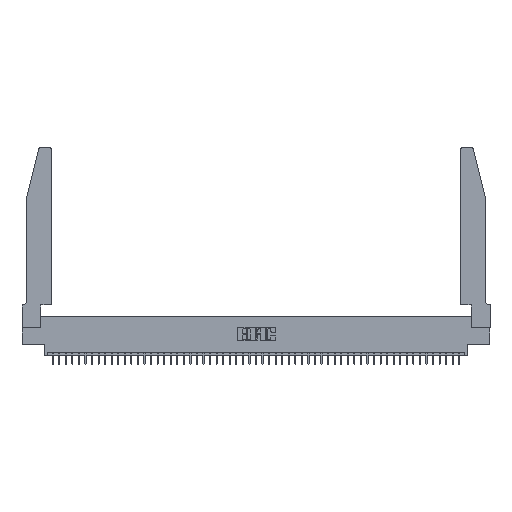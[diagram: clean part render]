
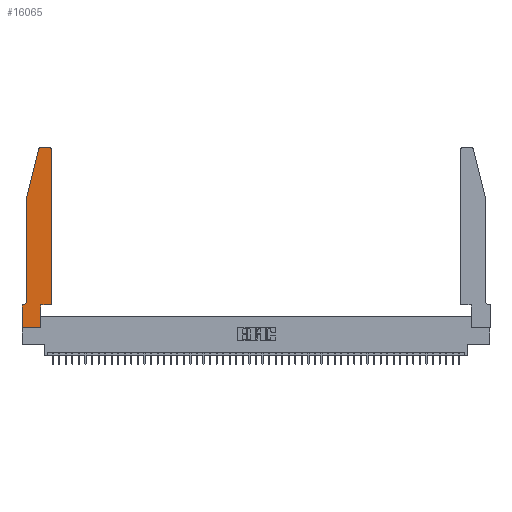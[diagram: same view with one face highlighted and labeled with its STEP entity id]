
A CAD part, top view. The second image highlights one B-rep face of the part: STEP entity #16065.
In plain terms, the highlighted planar face has unit normal (0, 0, 1).
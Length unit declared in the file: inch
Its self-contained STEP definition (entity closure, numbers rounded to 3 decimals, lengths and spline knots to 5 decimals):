
#1012 = CARTESIAN_POINT ( 'NONE',  ( 0.2865, 0., 0.37 ) ) ;
#1085 = ORIENTED_EDGE ( 'NONE', *, *, #47904, .T. ) ;
#1101 = VERTEX_POINT ( 'NONE', #1012 ) ;
#1142 = VECTOR ( 'NONE', #15414, 39.37008 ) ;
#1398 = DIRECTION ( 'NONE',  ( 1., 0., 0. ) ) ;
#1459 = CARTESIAN_POINT ( 'NONE',  ( 0.0755, 0.42, 0.37 ) ) ;
#1651 = CARTESIAN_POINT ( 'NONE',  ( 0.4505, 0.35, 0.37 ) ) ;
#1958 = EDGE_CURVE ( 'NONE', #10670, #44794, #8432, .T. ) ;
#1998 = CARTESIAN_POINT ( 'NONE',  ( 0., 0.35, 0.37 ) ) ;
#2457 = VERTEX_POINT ( 'NONE', #13750 ) ;
#3552 = CIRCLE ( 'NONE', #33524, 0.03 ) ;
#5090 = ORIENTED_EDGE ( 'NONE', *, *, #23087, .T. ) ;
#5956 = AXIS2_PLACEMENT_3D ( 'NONE', #39325, #47918, #23639 ) ;
#6470 = DIRECTION ( 'NONE',  ( 1., 0., 0. ) ) ;
#8432 = CIRCLE ( 'NONE', #5956, 0.07 ) ;
#8491 = LINE ( 'NONE', #9011, #38162 ) ;
#8721 = VECTOR ( 'NONE', #43241, 39.37008 ) ;
#9011 = CARTESIAN_POINT ( 'NONE',  ( 0.2865, 0.35, 0.37 ) ) ;
#9894 = EDGE_CURVE ( 'NONE', #2457, #12290, #41487, .T. ) ;
#10603 = LINE ( 'NONE', #13733, #8721 ) ;
#10623 = CARTESIAN_POINT ( 'NONE',  ( 0.0055, 0.35, 0.37 ) ) ;
#10670 = VERTEX_POINT ( 'NONE', #1459 ) ;
#10853 = VERTEX_POINT ( 'NONE', #34338 ) ;
#11432 = DIRECTION ( 'NONE',  ( 0., 0., 1. ) ) ;
#12290 = VERTEX_POINT ( 'NONE', #39814 ) ;
#12428 = LINE ( 'NONE', #24182, #37198 ) ;
#13638 = EDGE_CURVE ( 'NONE', #48304, #2457, #26218, .T. ) ;
#13733 = CARTESIAN_POINT ( 'NONE',  ( 0.0755, 0.35, 0.37 ) ) ;
#13750 = CARTESIAN_POINT ( 'NONE',  ( 0.4205, 2.75, 0.37 ) ) ;
#13987 = CARTESIAN_POINT ( 'NONE',  ( 0.0755, 2., 0.37 ) ) ;
#14022 = LINE ( 'NONE', #45903, #24774 ) ;
#14073 = VECTOR ( 'NONE', #1398, 39.37008 ) ;
#14960 = DIRECTION ( 'NONE',  ( 1., 0., 0. ) ) ;
#15414 = DIRECTION ( 'NONE',  ( 0., 1., 0. ) ) ;
#15603 = EDGE_CURVE ( 'NONE', #25376, #17163, #29401, .T. ) ;
#15662 = VERTEX_POINT ( 'NONE', #1998 ) ;
#15694 = EDGE_CURVE ( 'NONE', #44794, #15662, #10603, .T. ) ;
#16065 = ADVANCED_FACE ( 'NONE', ( #51011 ), #35059, .T. ) ;
#17163 = VERTEX_POINT ( 'NONE', #47922 ) ;
#17617 = ORIENTED_EDGE ( 'NONE', *, *, #15694, .T. ) ;
#17690 = ORIENTED_EDGE ( 'NONE', *, *, #28602, .T. ) ;
#18051 = VERTEX_POINT ( 'NONE', #48573 ) ;
#18813 = ORIENTED_EDGE ( 'NONE', *, *, #30267, .T. ) ;
#20901 = CARTESIAN_POINT ( 'NONE',  ( 0.25487, 2.72718, 0.37 ) ) ;
#21481 = EDGE_CURVE ( 'NONE', #50397, #18051, #45545, .T. ) ;
#22804 = CARTESIAN_POINT ( 'NONE',  ( 0., 0.35, 0.37 ) ) ;
#23087 = EDGE_CURVE ( 'NONE', #15662, #10853, #49726, .T. ) ;
#23639 = DIRECTION ( 'NONE',  ( -1., 0., 0. ) ) ;
#24182 = CARTESIAN_POINT ( 'NONE',  ( 0.0755, 2., 0.37 ) ) ;
#24774 = VECTOR ( 'NONE', #6470, 39.37008 ) ;
#24789 = ORIENTED_EDGE ( 'NONE', *, *, #13638, .T. ) ;
#25048 = ORIENTED_EDGE ( 'NONE', *, *, #47272, .T. ) ;
#25376 = VERTEX_POINT ( 'NONE', #20901 ) ;
#26218 = CIRCLE ( 'NONE', #50425, 0.03 ) ;
#26321 = CARTESIAN_POINT ( 'NONE',  ( 0.2605, 2.75, 0.37 ) ) ;
#28602 = EDGE_CURVE ( 'NONE', #12290, #25376, #3552, .T. ) ;
#29401 = LINE ( 'NONE', #13987, #33845 ) ;
#30267 = EDGE_CURVE ( 'NONE', #18051, #48304, #43903, .T. ) ;
#32164 = ORIENTED_EDGE ( 'NONE', *, *, #15603, .T. ) ;
#32226 = ORIENTED_EDGE ( 'NONE', *, *, #1958, .T. ) ;
#33518 = DIRECTION ( 'NONE',  ( 0., -1., 0. ) ) ;
#33524 = AXIS2_PLACEMENT_3D ( 'NONE', #38479, #34797, #37692 ) ;
#33845 = VECTOR ( 'NONE', #45611, 39.37008 ) ;
#34338 = CARTESIAN_POINT ( 'NONE',  ( 0., 0., 0.37 ) ) ;
#34670 = EDGE_LOOP ( 'NONE', ( #38746, #17690, #32164, #51001, #32226, #17617, #5090, #25048, #1085, #42284, #18813, #24789 ) ) ;
#34797 = DIRECTION ( 'NONE',  ( 0., 0., 1. ) ) ;
#34963 = VECTOR ( 'NONE', #33518, 39.37008 ) ;
#35059 = PLANE ( 'NONE',  #47213 ) ;
#35426 = DIRECTION ( 'NONE',  ( 0., -1., 0. ) ) ;
#37198 = VECTOR ( 'NONE', #35426, 39.37008 ) ;
#37291 = DIRECTION ( 'NONE',  ( -1., 0., 0. ) ) ;
#37692 = DIRECTION ( 'NONE',  ( 1., 0., 0. ) ) ;
#38162 = VECTOR ( 'NONE', #45064, 39.37008 ) ;
#38479 = CARTESIAN_POINT ( 'NONE',  ( 0.284, 2.72, 0.37 ) ) ;
#38746 = ORIENTED_EDGE ( 'NONE', *, *, #9894, .T. ) ;
#38997 = DIRECTION ( 'NONE',  ( 0., 0., 1. ) ) ;
#39325 = CARTESIAN_POINT ( 'NONE',  ( 0.0055, 0.42, 0.37 ) ) ;
#39814 = CARTESIAN_POINT ( 'NONE',  ( 0.284, 2.75, 0.37 ) ) ;
#39860 = CARTESIAN_POINT ( 'NONE',  ( 0.2865, 0.35, 0.37 ) ) ;
#41487 = LINE ( 'NONE', #26321, #41814 ) ;
#41814 = VECTOR ( 'NONE', #37291, 39.37008 ) ;
#42284 = ORIENTED_EDGE ( 'NONE', *, *, #21481, .T. ) ;
#43241 = DIRECTION ( 'NONE',  ( -1., 0., 0. ) ) ;
#43676 = EDGE_CURVE ( 'NONE', #17163, #10670, #12428, .T. ) ;
#43903 = LINE ( 'NONE', #50949, #1142 ) ;
#44794 = VERTEX_POINT ( 'NONE', #10623 ) ;
#44798 = CARTESIAN_POINT ( 'NONE',  ( 0., 0., 0.37 ) ) ;
#45064 = DIRECTION ( 'NONE',  ( 0., 1., 0. ) ) ;
#45545 = LINE ( 'NONE', #1651, #14073 ) ;
#45611 = DIRECTION ( 'NONE',  ( -0.239, -0.971, 0. ) ) ;
#45903 = CARTESIAN_POINT ( 'NONE',  ( 0., 0., 0.37 ) ) ;
#47213 = AXIS2_PLACEMENT_3D ( 'NONE', #22804, #38997, #14960 ) ;
#47218 = CARTESIAN_POINT ( 'NONE',  ( 0.4205, 2.72, 0.37 ) ) ;
#47272 = EDGE_CURVE ( 'NONE', #10853, #1101, #14022, .T. ) ;
#47722 = DIRECTION ( 'NONE',  ( 1., 0., 0. ) ) ;
#47904 = EDGE_CURVE ( 'NONE', #1101, #50397, #8491, .T. ) ;
#47918 = DIRECTION ( 'NONE',  ( 0., 0., -1. ) ) ;
#47922 = CARTESIAN_POINT ( 'NONE',  ( 0.0755, 2., 0.37 ) ) ;
#48304 = VERTEX_POINT ( 'NONE', #48590 ) ;
#48573 = CARTESIAN_POINT ( 'NONE',  ( 0.4505, 0.35, 0.37 ) ) ;
#48590 = CARTESIAN_POINT ( 'NONE',  ( 0.4505, 2.72, 0.37 ) ) ;
#49726 = LINE ( 'NONE', #44798, #34963 ) ;
#50397 = VERTEX_POINT ( 'NONE', #39860 ) ;
#50425 = AXIS2_PLACEMENT_3D ( 'NONE', #47218, #11432, #47722 ) ;
#50949 = CARTESIAN_POINT ( 'NONE',  ( 0.4505, 0.35, 0.37 ) ) ;
#51001 = ORIENTED_EDGE ( 'NONE', *, *, #43676, .T. ) ;
#51011 = FACE_OUTER_BOUND ( 'NONE', #34670, .T. ) ;
